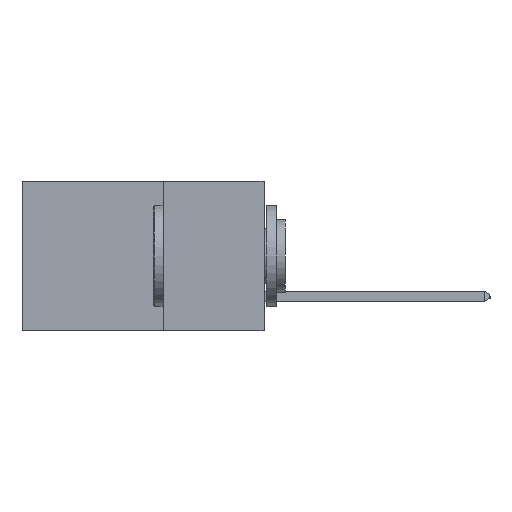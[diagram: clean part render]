
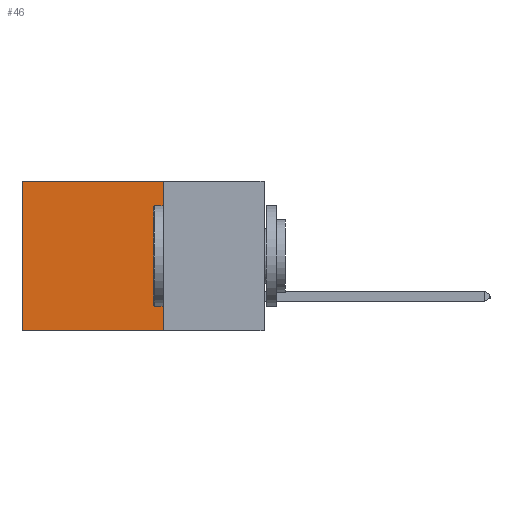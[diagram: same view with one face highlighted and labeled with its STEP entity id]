
A CAD part, left-side view. The second image highlights one B-rep face of the part: STEP entity #46.
In plain terms, the highlighted planar face has unit normal (-1, 0, 0).
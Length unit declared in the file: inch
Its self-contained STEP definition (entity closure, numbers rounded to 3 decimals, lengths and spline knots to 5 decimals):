
#46 = ADVANCED_FACE ( 'NONE', ( #21687 ), #12673, .F. ) ;
#286 = DIRECTION ( 'NONE',  ( 0., 1., 0. ) ) ;
#462 = CARTESIAN_POINT ( 'NONE',  ( 0.298, 0.25, -0.37 ) ) ;
#1684 = EDGE_LOOP ( 'NONE', ( #24224, #6552, #23501, #17914 ) ) ;
#1744 = CARTESIAN_POINT ( 'NONE',  ( 0.298, 0.25, -0.37 ) ) ;
#2210 = VERTEX_POINT ( 'NONE', #15346 ) ;
#2216 = VECTOR ( 'NONE', #286, 39.37008 ) ;
#2620 = LINE ( 'NONE', #25413, #18297 ) ;
#2856 = VECTOR ( 'NONE', #24160, 39.37008 ) ;
#3655 = CARTESIAN_POINT ( 'NONE',  ( 0.298, 0.6, 0. ) ) ;
#4177 = LINE ( 'NONE', #1744, #4807 ) ;
#4807 = VECTOR ( 'NONE', #7889, 39.37008 ) ;
#6552 = ORIENTED_EDGE ( 'NONE', *, *, #6887, .F. ) ;
#6887 = EDGE_CURVE ( 'NONE', #19958, #9105, #4177, .T. ) ;
#6923 = EDGE_CURVE ( 'NONE', #2210, #19958, #19149, .T. ) ;
#7702 = LINE ( 'NONE', #8491, #2216 ) ;
#7889 = DIRECTION ( 'NONE',  ( 0., 1., 0. ) ) ;
#8491 = CARTESIAN_POINT ( 'NONE',  ( 0.298, 0.25, 0. ) ) ;
#9105 = VERTEX_POINT ( 'NONE', #24359 ) ;
#9242 = DIRECTION ( 'NONE',  ( 0., 0., -1. ) ) ;
#10024 = CARTESIAN_POINT ( 'NONE',  ( 0.298, 0.25, 0. ) ) ;
#12602 = DIRECTION ( 'NONE',  ( 0., 0., -1. ) ) ;
#12673 = PLANE ( 'NONE',  #15713 ) ;
#13621 = VERTEX_POINT ( 'NONE', #3655 ) ;
#15346 = CARTESIAN_POINT ( 'NONE',  ( 0.298, 0.25, 0. ) ) ;
#15713 = AXIS2_PLACEMENT_3D ( 'NONE', #15949, #16431, #12602 ) ;
#15949 = CARTESIAN_POINT ( 'NONE',  ( 0.298, 0.25, 0. ) ) ;
#16431 = DIRECTION ( 'NONE',  ( 1., 0., 0. ) ) ;
#17914 = ORIENTED_EDGE ( 'NONE', *, *, #18529, .T. ) ;
#18297 = VECTOR ( 'NONE', #9242, 39.37008 ) ;
#18529 = EDGE_CURVE ( 'NONE', #2210, #13621, #7702, .T. ) ;
#19149 = LINE ( 'NONE', #10024, #2856 ) ;
#19958 = VERTEX_POINT ( 'NONE', #462 ) ;
#21687 = FACE_OUTER_BOUND ( 'NONE', #1684, .T. ) ;
#23501 = ORIENTED_EDGE ( 'NONE', *, *, #6923, .F. ) ;
#24160 = DIRECTION ( 'NONE',  ( 0., 0., -1. ) ) ;
#24224 = ORIENTED_EDGE ( 'NONE', *, *, #25701, .T. ) ;
#24359 = CARTESIAN_POINT ( 'NONE',  ( 0.298, 0.6, -0.37 ) ) ;
#25413 = CARTESIAN_POINT ( 'NONE',  ( 0.298, 0.6, 0. ) ) ;
#25701 = EDGE_CURVE ( 'NONE', #13621, #9105, #2620, .T. ) ;
